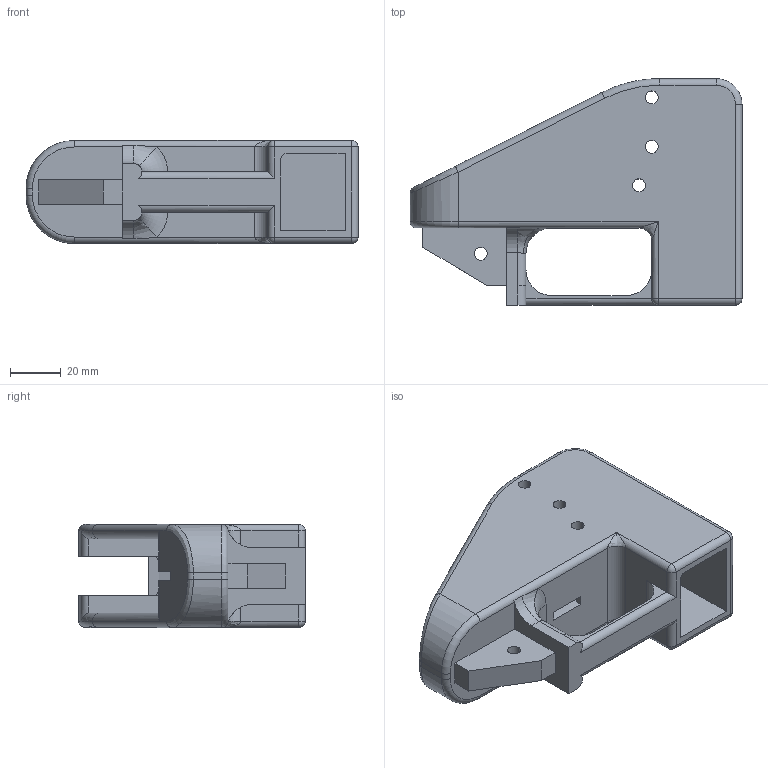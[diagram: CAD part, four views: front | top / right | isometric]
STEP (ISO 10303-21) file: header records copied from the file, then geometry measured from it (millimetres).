
FILE_DESCRIPTION (( 'STEP AP214' ), '1' );
FILE_NAME ('frame (no sn).STEP', '2013-05-27T22:44:53', ( 'Asher' ), ( '' ), 'SwSTEP 2.0', 'SolidWorks 2013', '' );
FILE_SCHEMA (( 'AUTOMOTIVE_DESIGN' ));
Length unit declared in the file: millimetre
Products named in the file (1): frame (no sn)
Bounding box: 130.94 x 89.31 x 40.64 mm (x, y, z)
Volume: 160087.2 mm3; surface area: 47527.4 mm2
Topology: 1 solids, 1 shells, 165 faces, 444 edges, 274 vertices
Faces by surface type: cylinder 69, plane 67, torus 17, bspline 6, sphere 4, cone 2
Entity records: 5582 total; most frequent: CARTESIAN_POINT 1388, DIRECTION 888, ORIENTED_EDGE 876, EDGE_CURVE 438, AXIS2_PLACEMENT_3D 320, VERTEX_POINT 274, VECTOR 248, LINE 248
